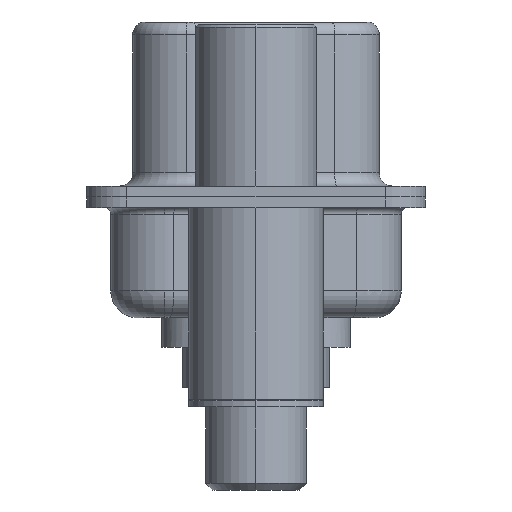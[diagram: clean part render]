
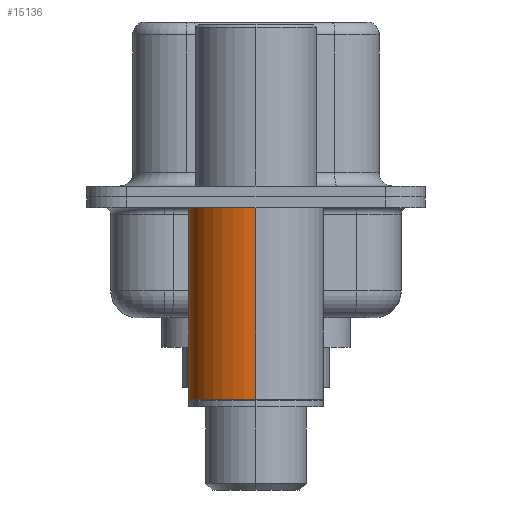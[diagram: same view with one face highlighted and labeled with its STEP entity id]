
A CAD part, left-side view. The second image highlights one B-rep face of the part: STEP entity #15136.
In plain terms, the highlighted cylindrical face has radius 2.5 mm (diameter 5 mm), a partial arc.
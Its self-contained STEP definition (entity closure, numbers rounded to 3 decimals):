
#544 = AXIS2_PLACEMENT_3D ( 'NONE', #11521, #5087, #3896 ) ;
#631 = VERTEX_POINT ( 'NONE', #12055 ) ;
#2102 = EDGE_CURVE ( 'NONE', #7141, #5437, #12101, .T. ) ;
#3061 = CARTESIAN_POINT ( 'NONE',  ( 0., 0., -7.525 ) ) ;
#3110 = LINE ( 'NONE', #10437, #3484 ) ;
#3484 = VECTOR ( 'NONE', #12986, 1000. ) ;
#3650 = CYLINDRICAL_SURFACE ( 'NONE', #544, 2.5 ) ;
#3896 = DIRECTION ( 'NONE',  ( 1., 0., 0. ) ) ;
#4262 = DIRECTION ( 'NONE',  ( 1., 0., 0. ) ) ;
#5087 = DIRECTION ( 'NONE',  ( 0., 0., 1. ) ) ;
#5186 = CARTESIAN_POINT ( 'NONE',  ( 0., 0., -0.4 ) ) ;
#5437 = VERTEX_POINT ( 'NONE', #6928 ) ;
#6195 = ORIENTED_EDGE ( 'NONE', *, *, #6272, .F. ) ;
#6272 = EDGE_CURVE ( 'NONE', #5437, #14390, #15573, .T. ) ;
#6392 = CARTESIAN_POINT ( 'NONE',  ( 2.5, 0., -7.525 ) ) ;
#6928 = CARTESIAN_POINT ( 'NONE',  ( 2.5, 0., -0.4 ) ) ;
#6989 = AXIS2_PLACEMENT_3D ( 'NONE', #5186, #7004, #15635 ) ;
#7004 = DIRECTION ( 'NONE',  ( 0., 0., 1. ) ) ;
#7141 = VERTEX_POINT ( 'NONE', #6392 ) ;
#8234 = ORIENTED_EDGE ( 'NONE', *, *, #2102, .F. ) ;
#8279 = ORIENTED_EDGE ( 'NONE', *, *, #10486, .T. ) ;
#8923 = AXIS2_PLACEMENT_3D ( 'NONE', #3061, #11891, #4262 ) ;
#9681 = EDGE_LOOP ( 'NONE', ( #12799, #8279, #6195, #8234 ) ) ;
#10437 = CARTESIAN_POINT ( 'NONE',  ( -2.5, 0., 0.581 ) ) ;
#10486 = EDGE_CURVE ( 'NONE', #631, #14390, #3110, .T. ) ;
#11300 = FACE_OUTER_BOUND ( 'NONE', #9681, .T. ) ;
#11521 = CARTESIAN_POINT ( 'NONE',  ( 0., 0., 0.581 ) ) ;
#11891 = DIRECTION ( 'NONE',  ( 0., 0., 1. ) ) ;
#12055 = CARTESIAN_POINT ( 'NONE',  ( -2.5, 0., -7.525 ) ) ;
#12101 = LINE ( 'NONE', #14308, #12492 ) ;
#12414 = EDGE_CURVE ( 'NONE', #7141, #631, #12537, .T. ) ;
#12492 = VECTOR ( 'NONE', #13590, 1000. ) ;
#12537 = CIRCLE ( 'NONE', #8923, 2.5 ) ;
#12799 = ORIENTED_EDGE ( 'NONE', *, *, #12414, .T. ) ;
#12986 = DIRECTION ( 'NONE',  ( 0., 0., 1. ) ) ;
#13590 = DIRECTION ( 'NONE',  ( 0., 0., 1. ) ) ;
#13822 = CARTESIAN_POINT ( 'NONE',  ( -2.5, 0., -0.4 ) ) ;
#14308 = CARTESIAN_POINT ( 'NONE',  ( 2.5, 0., 0.581 ) ) ;
#14390 = VERTEX_POINT ( 'NONE', #13822 ) ;
#15136 = ADVANCED_FACE ( 'NONE', ( #11300 ), #3650, .T. ) ;
#15573 = CIRCLE ( 'NONE', #6989, 2.5 ) ;
#15635 = DIRECTION ( 'NONE',  ( 1., 0., 0. ) ) ;
